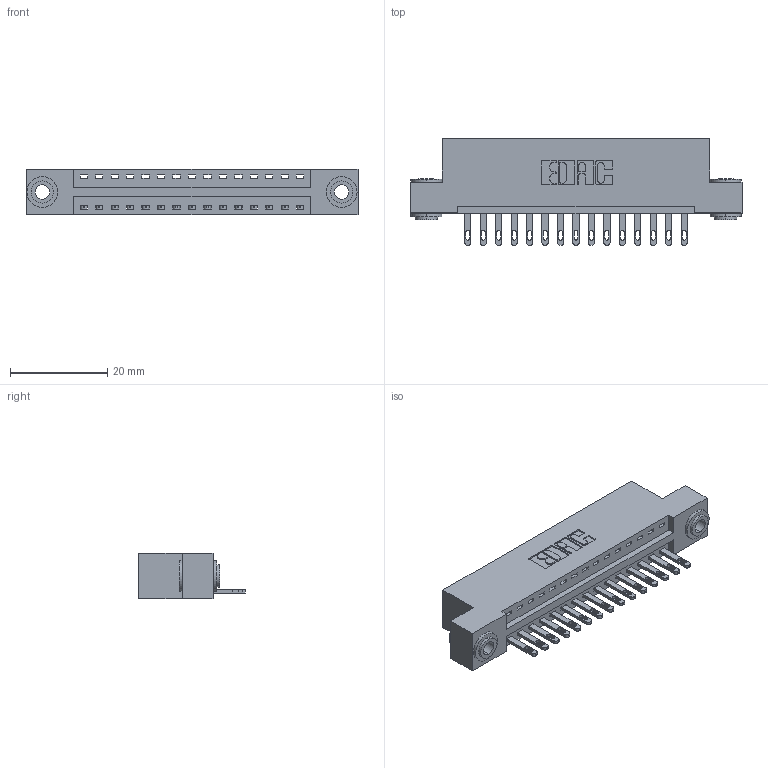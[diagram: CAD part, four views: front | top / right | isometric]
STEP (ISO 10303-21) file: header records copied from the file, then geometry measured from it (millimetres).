
FILE_DESCRIPTION (( 'STEP AP203' ), '1' );
FILE_NAME ('896-015-500-103.STEP', '2021-07-27T15:24:50', ( '' ), ( '' ), 'SwSTEP 2.0', 'SolidWorks 2020', '' );
FILE_SCHEMA (( 'CONFIG_CONTROL_DESIGN' ));
Length unit declared in the file: inch
Products named in the file (4): 345-250-002_345-250-002-102; 345-292-001_345-293-100; 896-015-500-103; 846 Part_Flush Mounting Lugs - 0.156 Dia-TH
Assembly tree (18 placements, depth 2):
  896-015-500-103
    846 Part_Flush Mounting Lugs - 0.156 Dia-TH
    345-292-001_345-293-100  x15
    345-250-002_345-250-002-102  x2
Bounding box: 68.2 x 21.84 x 9.4 mm (x, y, z)
Volume: 6370.8 mm3; surface area: 7925.5 mm2
Topology: 18 solids, 18 shells, 970 faces, 2925 edges, 1946 vertices
Faces by surface type: plane 596, cylinder 366, cone 8
Entity records: 13524 total; most frequent: CARTESIAN_POINT 2304, ORIENTED_EDGE 2246, DIRECTION 2099, EDGE_CURVE 1123, LINE 903, VECTOR 903, VERTEX_POINT 746, AXIS2_PLACEMENT_3D 598
